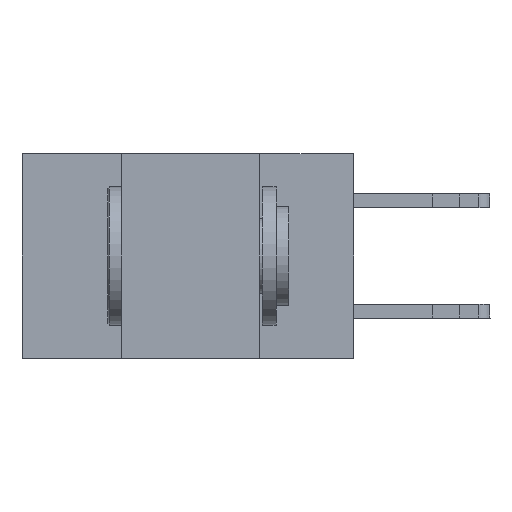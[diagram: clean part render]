
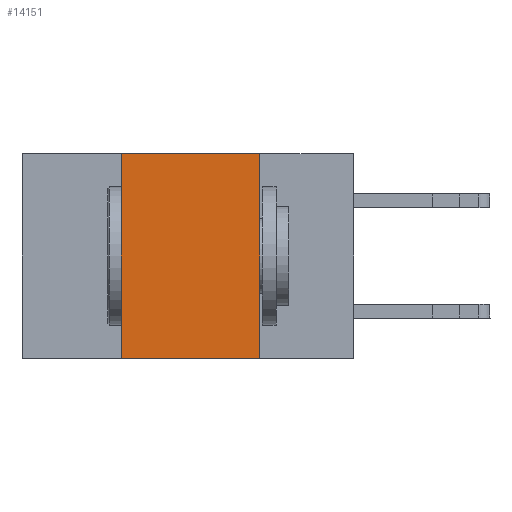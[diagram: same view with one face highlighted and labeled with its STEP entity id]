
A CAD part, left-side view. The second image highlights one B-rep face of the part: STEP entity #14151.
In plain terms, the highlighted planar face has unit normal (-1, 0, 0).
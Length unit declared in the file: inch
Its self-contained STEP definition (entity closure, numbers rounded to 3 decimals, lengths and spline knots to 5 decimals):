
#484 = CARTESIAN_POINT ( 'NONE',  ( 0., 0.6, -0.37 ) ) ;
#1155 = CARTESIAN_POINT ( 'NONE',  ( 0., 0.6, 0. ) ) ;
#2154 = CARTESIAN_POINT ( 'NONE',  ( 0., 0.17, 0. ) ) ;
#3077 = DIRECTION ( 'NONE',  ( 0., 0., 1. ) ) ;
#3839 = LINE ( 'NONE', #15568, #11022 ) ;
#4170 = LINE ( 'NONE', #1155, #9072 ) ;
#4195 = VERTEX_POINT ( 'NONE', #17830 ) ;
#4292 = EDGE_CURVE ( 'NONE', #7160, #6486, #7786, .T. ) ;
#6486 = VERTEX_POINT ( 'NONE', #14373 ) ;
#7160 = VERTEX_POINT ( 'NONE', #19616 ) ;
#7713 = LINE ( 'NONE', #12004, #8358 ) ;
#7786 = LINE ( 'NONE', #484, #13645 ) ;
#8358 = VECTOR ( 'NONE', #26688, 39.37008 ) ;
#9072 = VECTOR ( 'NONE', #13919, 39.37008 ) ;
#9095 = ORIENTED_EDGE ( 'NONE', *, *, #4292, .T. ) ;
#9453 = CARTESIAN_POINT ( 'NONE',  ( 0., 0.6, 0. ) ) ;
#9634 = VERTEX_POINT ( 'NONE', #2154 ) ;
#11022 = VECTOR ( 'NONE', #3077, 39.37008 ) ;
#11349 = EDGE_CURVE ( 'NONE', #4195, #9634, #4170, .T. ) ;
#11538 = DIRECTION ( 'NONE',  ( 1., 0., 0. ) ) ;
#12004 = CARTESIAN_POINT ( 'NONE',  ( 0., 0.17, 0. ) ) ;
#12824 = ORIENTED_EDGE ( 'NONE', *, *, #14607, .F. ) ;
#13005 = EDGE_CURVE ( 'NONE', #7160, #4195, #3839, .T. ) ;
#13248 = DIRECTION ( 'NONE',  ( 0., -1., 0. ) ) ;
#13645 = VECTOR ( 'NONE', #13248, 39.37008 ) ;
#13725 = PLANE ( 'NONE',  #17490 ) ;
#13919 = DIRECTION ( 'NONE',  ( 0., -1., 0. ) ) ;
#14151 = ADVANCED_FACE ( 'NONE', ( #16596 ), #13725, .F. ) ;
#14373 = CARTESIAN_POINT ( 'NONE',  ( 0., 0.17, -0.37 ) ) ;
#14607 = EDGE_CURVE ( 'NONE', #9634, #6486, #7713, .T. ) ;
#15568 = CARTESIAN_POINT ( 'NONE',  ( 0., 0.42, 0. ) ) ;
#16596 = FACE_OUTER_BOUND ( 'NONE', #19321, .T. ) ;
#17490 = AXIS2_PLACEMENT_3D ( 'NONE', #9453, #11538, #26311 ) ;
#17830 = CARTESIAN_POINT ( 'NONE',  ( 0., 0.42, 0. ) ) ;
#19321 = EDGE_LOOP ( 'NONE', ( #12824, #24638, #21394, #9095 ) ) ;
#19616 = CARTESIAN_POINT ( 'NONE',  ( 0., 0.42, -0.37 ) ) ;
#21394 = ORIENTED_EDGE ( 'NONE', *, *, #13005, .F. ) ;
#24638 = ORIENTED_EDGE ( 'NONE', *, *, #11349, .F. ) ;
#26311 = DIRECTION ( 'NONE',  ( 0., 0., -1. ) ) ;
#26688 = DIRECTION ( 'NONE',  ( 0., 0., -1. ) ) ;
